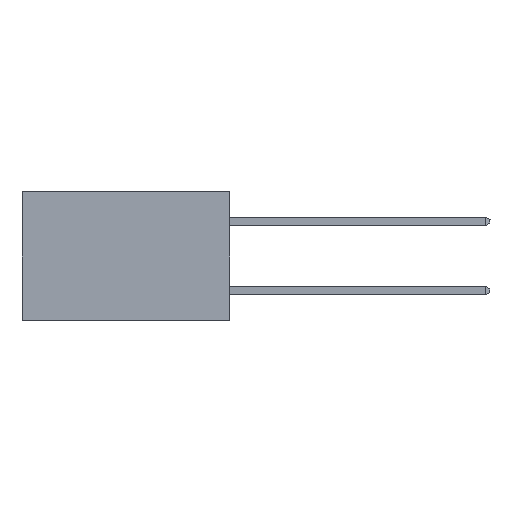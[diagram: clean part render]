
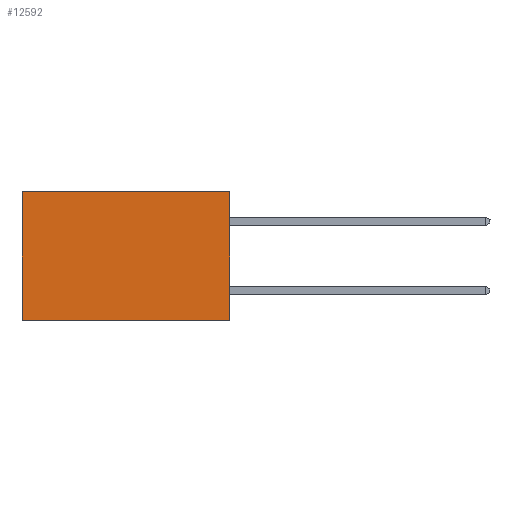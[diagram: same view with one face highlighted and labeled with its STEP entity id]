
A CAD part, left-side view. The second image highlights one B-rep face of the part: STEP entity #12592.
In plain terms, the highlighted planar face has unit normal (-1, 0, 0).
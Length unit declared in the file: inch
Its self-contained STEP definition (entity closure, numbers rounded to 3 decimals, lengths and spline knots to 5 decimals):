
#253 = ORIENTED_EDGE ( 'NONE', *, *, #13606, .F. ) ;
#908 = LINE ( 'NONE', #9470, #10097 ) ;
#1738 = ORIENTED_EDGE ( 'NONE', *, *, #10554, .T. ) ;
#2013 = EDGE_CURVE ( 'NONE', #2902, #8147, #8871, .T. ) ;
#2093 = VERTEX_POINT ( 'NONE', #8184 ) ;
#2902 = VERTEX_POINT ( 'NONE', #17542 ) ;
#4445 = CARTESIAN_POINT ( 'NONE',  ( 0.2615, 0., -0.37 ) ) ;
#5003 = CARTESIAN_POINT ( 'NONE',  ( 0.2615, 0., 0. ) ) ;
#5713 = CARTESIAN_POINT ( 'NONE',  ( 0.2615, 0.6, -0.37 ) ) ;
#6947 = VERTEX_POINT ( 'NONE', #5003 ) ;
#7387 = EDGE_CURVE ( 'NONE', #2093, #8147, #908, .T. ) ;
#8131 = DIRECTION ( 'NONE',  ( 0., 1., 0. ) ) ;
#8147 = VERTEX_POINT ( 'NONE', #5713 ) ;
#8184 = CARTESIAN_POINT ( 'NONE',  ( 0.2615, 0.6, 0. ) ) ;
#8409 = DIRECTION ( 'NONE',  ( 0., 0., -1. ) ) ;
#8871 = LINE ( 'NONE', #4445, #12532 ) ;
#9470 = CARTESIAN_POINT ( 'NONE',  ( 0.2615, 0.6, -0.37 ) ) ;
#9921 = LINE ( 'NONE', #15645, #13567 ) ;
#10097 = VECTOR ( 'NONE', #12366, 39.37008 ) ;
#10554 = EDGE_CURVE ( 'NONE', #6947, #2093, #18172, .T. ) ;
#11024 = DIRECTION ( 'NONE',  ( 1., 0., 0. ) ) ;
#12260 = ORIENTED_EDGE ( 'NONE', *, *, #2013, .F. ) ;
#12366 = DIRECTION ( 'NONE',  ( 0., 0., -1. ) ) ;
#12532 = VECTOR ( 'NONE', #14595, 39.37008 ) ;
#12592 = ADVANCED_FACE ( 'NONE', ( #15541 ), #13844, .F. ) ;
#12834 = DIRECTION ( 'NONE',  ( 0., 0., -1. ) ) ;
#13567 = VECTOR ( 'NONE', #12834, 39.37008 ) ;
#13606 = EDGE_CURVE ( 'NONE', #6947, #2902, #9921, .T. ) ;
#13844 = PLANE ( 'NONE',  #15942 ) ;
#14594 = EDGE_LOOP ( 'NONE', ( #17384, #12260, #253, #1738 ) ) ;
#14595 = DIRECTION ( 'NONE',  ( 0., 1., 0. ) ) ;
#15349 = CARTESIAN_POINT ( 'NONE',  ( 0.2615, 0., -0.37 ) ) ;
#15541 = FACE_OUTER_BOUND ( 'NONE', #14594, .T. ) ;
#15645 = CARTESIAN_POINT ( 'NONE',  ( 0.2615, 0., -0.37 ) ) ;
#15942 = AXIS2_PLACEMENT_3D ( 'NONE', #15349, #11024, #8409 ) ;
#16953 = CARTESIAN_POINT ( 'NONE',  ( 0.2615, 0., 0. ) ) ;
#17384 = ORIENTED_EDGE ( 'NONE', *, *, #7387, .T. ) ;
#17542 = CARTESIAN_POINT ( 'NONE',  ( 0.2615, 0., -0.37 ) ) ;
#18172 = LINE ( 'NONE', #16953, #18301 ) ;
#18301 = VECTOR ( 'NONE', #8131, 39.37008 ) ;
